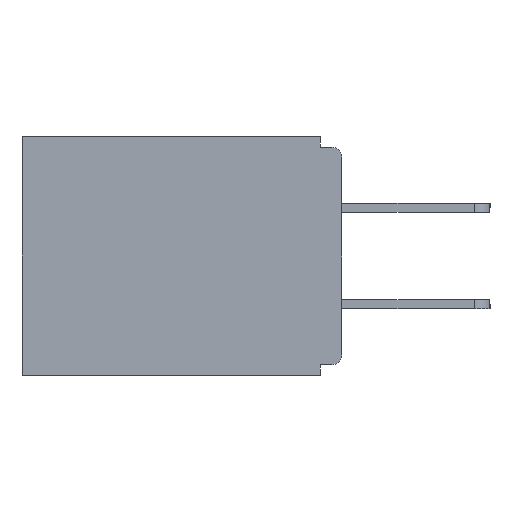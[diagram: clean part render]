
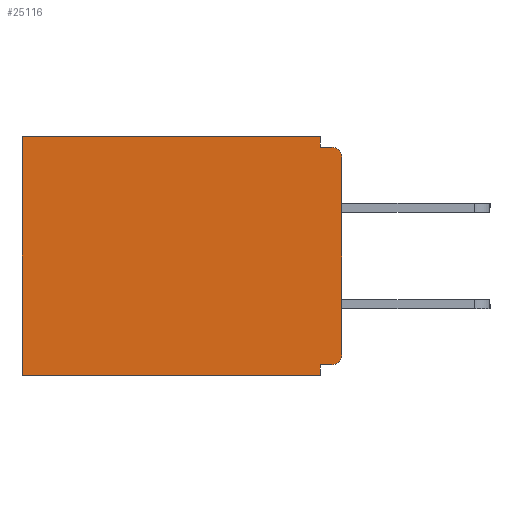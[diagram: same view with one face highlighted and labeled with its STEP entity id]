
A CAD part, left-side view. The second image highlights one B-rep face of the part: STEP entity #25116.
In plain terms, the highlighted planar face has unit normal (-1, 0, 0).
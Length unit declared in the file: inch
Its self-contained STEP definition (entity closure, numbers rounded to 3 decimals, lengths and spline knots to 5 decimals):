
#67 = DIRECTION ( 'NONE',  ( -1., 0., 0. ) ) ;
#351 = EDGE_CURVE ( 'NONE', #10469, #18375, #456, .T. ) ;
#456 = LINE ( 'NONE', #23685, #12749 ) ;
#646 = LINE ( 'NONE', #22679, #11672 ) ;
#1023 = DIRECTION ( 'NONE',  ( 1., 0., 0. ) ) ;
#1534 = ORIENTED_EDGE ( 'NONE', *, *, #21078, .T. ) ;
#1818 = EDGE_CURVE ( 'NONE', #20375, #21336, #2027, .T. ) ;
#2027 = CIRCLE ( 'NONE', #2284, 0.015 ) ;
#2284 = AXIS2_PLACEMENT_3D ( 'NONE', #17904, #24020, #13857 ) ;
#2836 = LINE ( 'NONE', #13243, #19286 ) ;
#2846 = CARTESIAN_POINT ( 'NONE',  ( 0.298, 0.031, -0.343 ) ) ;
#3085 = VECTOR ( 'NONE', #17696, 39.37008 ) ;
#3693 = ORIENTED_EDGE ( 'NONE', *, *, #13880, .F. ) ;
#3831 = CARTESIAN_POINT ( 'NONE',  ( 0.298, 0., -0.343 ) ) ;
#5617 = EDGE_CURVE ( 'NONE', #8341, #6273, #24303, .T. ) ;
#5646 = EDGE_CURVE ( 'NONE', #14628, #6273, #646, .T. ) ;
#5865 = VECTOR ( 'NONE', #14619, 39.37008 ) ;
#5916 = CARTESIAN_POINT ( 'NONE',  ( 0.298, 0.031, -0.328 ) ) ;
#6273 = VERTEX_POINT ( 'NONE', #12987 ) ;
#6950 = CARTESIAN_POINT ( 'NONE',  ( 0.298, 0., -0.313 ) ) ;
#7364 = AXIS2_PLACEMENT_3D ( 'NONE', #21514, #1023, #25637 ) ;
#7667 = VERTEX_POINT ( 'NONE', #5916 ) ;
#7669 = VERTEX_POINT ( 'NONE', #24210 ) ;
#8202 = LINE ( 'NONE', #2846, #24001 ) ;
#8341 = VERTEX_POINT ( 'NONE', #24488 ) ;
#8608 = LINE ( 'NONE', #15646, #3085 ) ;
#8742 = ORIENTED_EDGE ( 'NONE', *, *, #5617, .T. ) ;
#10145 = ORIENTED_EDGE ( 'NONE', *, *, #10927, .F. ) ;
#10469 = VERTEX_POINT ( 'NONE', #18715 ) ;
#10485 = AXIS2_PLACEMENT_3D ( 'NONE', #12369, #67, #16397 ) ;
#10927 = EDGE_CURVE ( 'NONE', #7667, #16322, #26282, .T. ) ;
#11351 = PLANE ( 'NONE',  #7364 ) ;
#11396 = LINE ( 'NONE', #3831, #21702 ) ;
#11672 = VECTOR ( 'NONE', #20483, 39.37008 ) ;
#11752 = VECTOR ( 'NONE', #16074, 39.37008 ) ;
#12369 = CARTESIAN_POINT ( 'NONE',  ( 0.298, 0.015, -0.03 ) ) ;
#12558 = CARTESIAN_POINT ( 'NONE',  ( 0.298, 0.031, -0.343 ) ) ;
#12749 = VECTOR ( 'NONE', #15410, 39.37008 ) ;
#12987 = CARTESIAN_POINT ( 'NONE',  ( 0.298, 0.015, -0.015 ) ) ;
#13243 = CARTESIAN_POINT ( 'NONE',  ( 0.298, 0., 0. ) ) ;
#13857 = DIRECTION ( 'NONE',  ( 0., 0., -1. ) ) ;
#13880 = EDGE_CURVE ( 'NONE', #8341, #21336, #2836, .T. ) ;
#14619 = DIRECTION ( 'NONE',  ( 0., 0., -1. ) ) ;
#14628 = VERTEX_POINT ( 'NONE', #24198 ) ;
#15410 = DIRECTION ( 'NONE',  ( 0., 0., -1. ) ) ;
#15646 = CARTESIAN_POINT ( 'NONE',  ( 0.298, 0., 0. ) ) ;
#16074 = DIRECTION ( 'NONE',  ( 0., 1., 0. ) ) ;
#16322 = VERTEX_POINT ( 'NONE', #16434 ) ;
#16397 = DIRECTION ( 'NONE',  ( 0., 0., -1. ) ) ;
#16434 = CARTESIAN_POINT ( 'NONE',  ( 0.298, 0.031, -0.343 ) ) ;
#16843 = EDGE_CURVE ( 'NONE', #16322, #18375, #11396, .T. ) ;
#16870 = ORIENTED_EDGE ( 'NONE', *, *, #351, .T. ) ;
#17198 = LINE ( 'NONE', #24247, #11752 ) ;
#17255 = DIRECTION ( 'NONE',  ( 0., 0., -1. ) ) ;
#17696 = DIRECTION ( 'NONE',  ( 0., 1., 0. ) ) ;
#17904 = CARTESIAN_POINT ( 'NONE',  ( 0.298, 0.015, -0.313 ) ) ;
#18375 = VERTEX_POINT ( 'NONE', #24153 ) ;
#18715 = CARTESIAN_POINT ( 'NONE',  ( 0.298, 0.46, 0. ) ) ;
#19286 = VECTOR ( 'NONE', #25860, 39.37008 ) ;
#19695 = FACE_OUTER_BOUND ( 'NONE', #23436, .T. ) ;
#20162 = ORIENTED_EDGE ( 'NONE', *, *, #5646, .F. ) ;
#20238 = ORIENTED_EDGE ( 'NONE', *, *, #23909, .F. ) ;
#20375 = VERTEX_POINT ( 'NONE', #22328 ) ;
#20483 = DIRECTION ( 'NONE',  ( 0., -1., 0. ) ) ;
#21078 = EDGE_CURVE ( 'NONE', #7669, #10469, #8608, .T. ) ;
#21336 = VERTEX_POINT ( 'NONE', #6950 ) ;
#21514 = CARTESIAN_POINT ( 'NONE',  ( 0.298, 0., 0. ) ) ;
#21527 = ORIENTED_EDGE ( 'NONE', *, *, #16843, .F. ) ;
#21702 = VECTOR ( 'NONE', #22435, 39.37008 ) ;
#22328 = CARTESIAN_POINT ( 'NONE',  ( 0.298, 0.015, -0.328 ) ) ;
#22435 = DIRECTION ( 'NONE',  ( 0., 1., 0. ) ) ;
#22679 = CARTESIAN_POINT ( 'NONE',  ( 0.298, 0., -0.015 ) ) ;
#22897 = EDGE_CURVE ( 'NONE', #20375, #7667, #17198, .T. ) ;
#23436 = EDGE_LOOP ( 'NONE', ( #8742, #20162, #20238, #1534, #16870, #21527, #10145, #24854, #26352, #3693 ) ) ;
#23685 = CARTESIAN_POINT ( 'NONE',  ( 0.298, 0.46, 0. ) ) ;
#23909 = EDGE_CURVE ( 'NONE', #7669, #14628, #8202, .T. ) ;
#24001 = VECTOR ( 'NONE', #17255, 39.37008 ) ;
#24020 = DIRECTION ( 'NONE',  ( -1., 0., 0. ) ) ;
#24153 = CARTESIAN_POINT ( 'NONE',  ( 0.298, 0.46, -0.343 ) ) ;
#24198 = CARTESIAN_POINT ( 'NONE',  ( 0.298, 0.031, -0.015 ) ) ;
#24210 = CARTESIAN_POINT ( 'NONE',  ( 0.298, 0.031, 0. ) ) ;
#24247 = CARTESIAN_POINT ( 'NONE',  ( 0.298, 0., -0.328 ) ) ;
#24303 = CIRCLE ( 'NONE', #10485, 0.015 ) ;
#24488 = CARTESIAN_POINT ( 'NONE',  ( 0.298, 0., -0.03 ) ) ;
#24854 = ORIENTED_EDGE ( 'NONE', *, *, #22897, .F. ) ;
#25116 = ADVANCED_FACE ( 'NONE', ( #19695 ), #11351, .F. ) ;
#25637 = DIRECTION ( 'NONE',  ( 0., 0., -1. ) ) ;
#25860 = DIRECTION ( 'NONE',  ( 0., 0., -1. ) ) ;
#26282 = LINE ( 'NONE', #12558, #5865 ) ;
#26352 = ORIENTED_EDGE ( 'NONE', *, *, #1818, .T. ) ;
